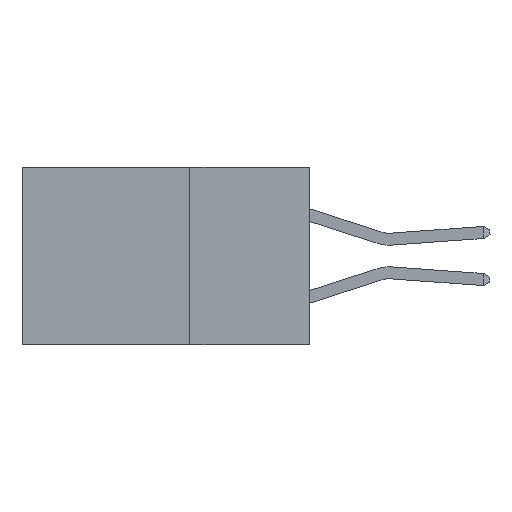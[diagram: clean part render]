
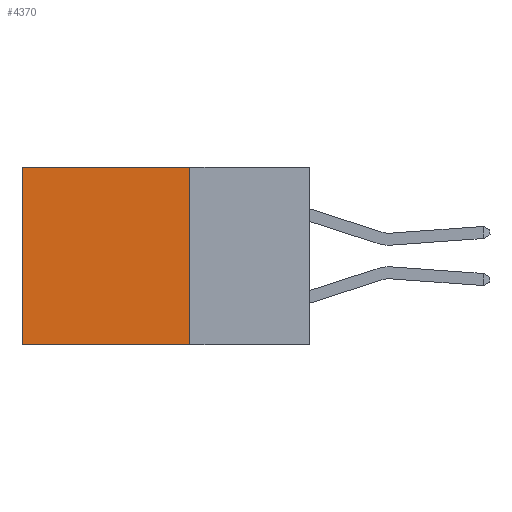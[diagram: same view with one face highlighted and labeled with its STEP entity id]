
A CAD part, left-side view. The second image highlights one B-rep face of the part: STEP entity #4370.
In plain terms, the highlighted planar face has unit normal (-1, 0, 0).
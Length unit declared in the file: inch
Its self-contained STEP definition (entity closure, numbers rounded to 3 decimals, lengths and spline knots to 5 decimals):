
#1052 = CARTESIAN_POINT ( 'NONE',  ( 0.298, 0.6, 0. ) ) ;
#1235 = DIRECTION ( 'NONE',  ( 0., 1., 0. ) ) ;
#1898 = EDGE_LOOP ( 'NONE', ( #6218, #5207, #6610, #10262 ) ) ;
#2058 = VECTOR ( 'NONE', #6042, 39.37008 ) ;
#2505 = LINE ( 'NONE', #11223, #12023 ) ;
#3219 = EDGE_CURVE ( 'NONE', #3933, #10804, #10460, .T. ) ;
#3671 = CARTESIAN_POINT ( 'NONE',  ( 0.298, 0.25, 0. ) ) ;
#3933 = VERTEX_POINT ( 'NONE', #1052 ) ;
#4370 = ADVANCED_FACE ( 'NONE', ( #8470 ), #6700, .F. ) ;
#4654 = VERTEX_POINT ( 'NONE', #13379 ) ;
#5207 = ORIENTED_EDGE ( 'NONE', *, *, #6220, .F. ) ;
#5425 = LINE ( 'NONE', #3671, #2058 ) ;
#5546 = CARTESIAN_POINT ( 'NONE',  ( 0.298, 0.25, 0. ) ) ;
#6042 = DIRECTION ( 'NONE',  ( 0., 1., 0. ) ) ;
#6218 = ORIENTED_EDGE ( 'NONE', *, *, #3219, .T. ) ;
#6220 = EDGE_CURVE ( 'NONE', #4654, #10804, #14176, .T. ) ;
#6610 = ORIENTED_EDGE ( 'NONE', *, *, #15309, .F. ) ;
#6700 = PLANE ( 'NONE',  #10146 ) ;
#6937 = CARTESIAN_POINT ( 'NONE',  ( 0.298, 0.6, 0. ) ) ;
#7847 = DIRECTION ( 'NONE',  ( 0., 0., -1. ) ) ;
#8470 = FACE_OUTER_BOUND ( 'NONE', #1898, .T. ) ;
#8635 = CARTESIAN_POINT ( 'NONE',  ( 0.298, 0.25, -0.37 ) ) ;
#10146 = AXIS2_PLACEMENT_3D ( 'NONE', #5546, #14921, #7847 ) ;
#10262 = ORIENTED_EDGE ( 'NONE', *, *, #11681, .T. ) ;
#10460 = LINE ( 'NONE', #6937, #12850 ) ;
#10469 = DIRECTION ( 'NONE',  ( 0., 0., -1. ) ) ;
#10804 = VERTEX_POINT ( 'NONE', #12990 ) ;
#11028 = VECTOR ( 'NONE', #1235, 39.37008 ) ;
#11171 = DIRECTION ( 'NONE',  ( 0., 0., -1. ) ) ;
#11223 = CARTESIAN_POINT ( 'NONE',  ( 0.298, 0.25, 0. ) ) ;
#11422 = CARTESIAN_POINT ( 'NONE',  ( 0.298, 0.25, 0. ) ) ;
#11681 = EDGE_CURVE ( 'NONE', #15459, #3933, #5425, .T. ) ;
#12023 = VECTOR ( 'NONE', #11171, 39.37008 ) ;
#12850 = VECTOR ( 'NONE', #10469, 39.37008 ) ;
#12990 = CARTESIAN_POINT ( 'NONE',  ( 0.298, 0.6, -0.37 ) ) ;
#13379 = CARTESIAN_POINT ( 'NONE',  ( 0.298, 0.25, -0.37 ) ) ;
#14176 = LINE ( 'NONE', #8635, #11028 ) ;
#14921 = DIRECTION ( 'NONE',  ( 1., 0., 0. ) ) ;
#15309 = EDGE_CURVE ( 'NONE', #15459, #4654, #2505, .T. ) ;
#15459 = VERTEX_POINT ( 'NONE', #11422 ) ;
